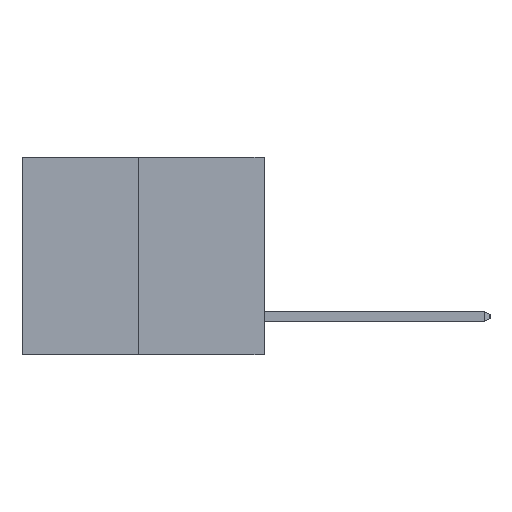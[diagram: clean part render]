
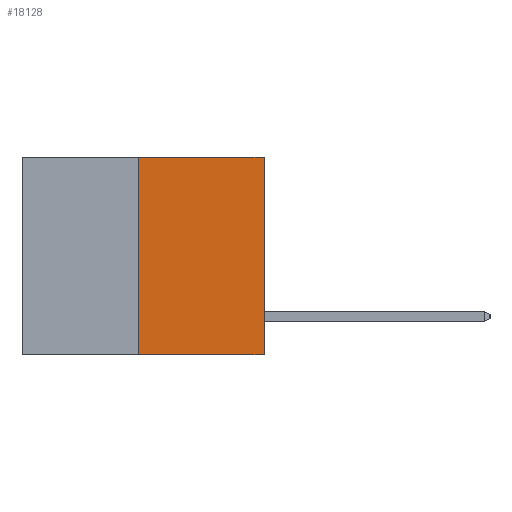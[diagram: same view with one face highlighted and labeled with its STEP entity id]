
A CAD part, left-side view. The second image highlights one B-rep face of the part: STEP entity #18128.
In plain terms, the highlighted planar face has unit normal (-1, 0, 0).
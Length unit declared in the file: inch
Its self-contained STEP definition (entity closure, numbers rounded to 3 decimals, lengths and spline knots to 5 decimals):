
#1140 = EDGE_CURVE ( 'NONE', #22509, #28499, #24951, .T. ) ;
#1517 = VECTOR ( 'NONE', #22203, 39.37008 ) ;
#2156 = VECTOR ( 'NONE', #7741, 39.37008 ) ;
#3413 = AXIS2_PLACEMENT_3D ( 'NONE', #5266, #9761, #19032 ) ;
#3710 = LINE ( 'NONE', #10742, #1517 ) ;
#5266 = CARTESIAN_POINT ( 'NONE',  ( 0., 0.6, 0. ) ) ;
#5775 = LINE ( 'NONE', #16893, #2156 ) ;
#6311 = EDGE_CURVE ( 'NONE', #22509, #25405, #5775, .T. ) ;
#7260 = CARTESIAN_POINT ( 'NONE',  ( 0., 0., 0. ) ) ;
#7741 = DIRECTION ( 'NONE',  ( 0., -1., 0. ) ) ;
#8416 = FACE_OUTER_BOUND ( 'NONE', #22994, .T. ) ;
#8830 = ORIENTED_EDGE ( 'NONE', *, *, #18895, .T. ) ;
#9761 = DIRECTION ( 'NONE',  ( 1., 0., 0. ) ) ;
#10288 = DIRECTION ( 'NONE',  ( 0., -1., 0. ) ) ;
#10742 = CARTESIAN_POINT ( 'NONE',  ( 0., 0., 0. ) ) ;
#12022 = VECTOR ( 'NONE', #19849, 39.37008 ) ;
#12426 = CARTESIAN_POINT ( 'NONE',  ( 0., 0.6, 0. ) ) ;
#12629 = CARTESIAN_POINT ( 'NONE',  ( 0., 0.312, -0.49 ) ) ;
#13275 = LINE ( 'NONE', #12426, #21504 ) ;
#15434 = CARTESIAN_POINT ( 'NONE',  ( 0., 0.312, -0.49 ) ) ;
#15853 = ORIENTED_EDGE ( 'NONE', *, *, #6311, .T. ) ;
#15906 = CARTESIAN_POINT ( 'NONE',  ( 0., 0.312, 0. ) ) ;
#16893 = CARTESIAN_POINT ( 'NONE',  ( 0., 0.6, -0.49 ) ) ;
#18128 = ADVANCED_FACE ( 'NONE', ( #8416 ), #23629, .F. ) ;
#18895 = EDGE_CURVE ( 'NONE', #25405, #29203, #3710, .T. ) ;
#19032 = DIRECTION ( 'NONE',  ( 0., 0., -1. ) ) ;
#19849 = DIRECTION ( 'NONE',  ( 0., 0., 1. ) ) ;
#21504 = VECTOR ( 'NONE', #10288, 39.37008 ) ;
#22203 = DIRECTION ( 'NONE',  ( 0., 0., 1. ) ) ;
#22509 = VERTEX_POINT ( 'NONE', #15434 ) ;
#22994 = EDGE_LOOP ( 'NONE', ( #27854, #15853, #8830, #28363 ) ) ;
#23629 = PLANE ( 'NONE',  #3413 ) ;
#24951 = LINE ( 'NONE', #12629, #12022 ) ;
#24960 = CARTESIAN_POINT ( 'NONE',  ( 0., 0., -0.49 ) ) ;
#25405 = VERTEX_POINT ( 'NONE', #24960 ) ;
#26072 = EDGE_CURVE ( 'NONE', #28499, #29203, #13275, .T. ) ;
#27854 = ORIENTED_EDGE ( 'NONE', *, *, #1140, .F. ) ;
#28363 = ORIENTED_EDGE ( 'NONE', *, *, #26072, .F. ) ;
#28499 = VERTEX_POINT ( 'NONE', #15906 ) ;
#29203 = VERTEX_POINT ( 'NONE', #7260 ) ;
